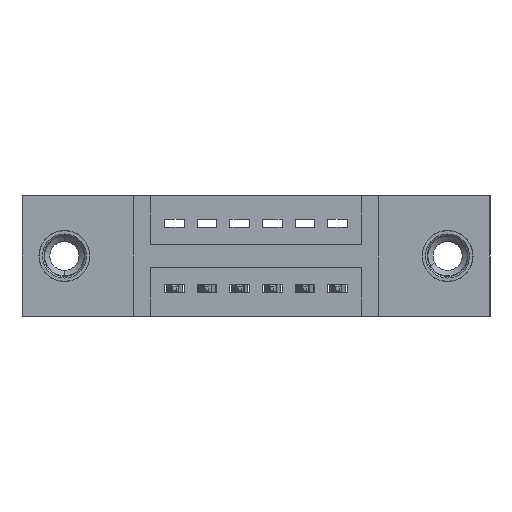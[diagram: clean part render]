
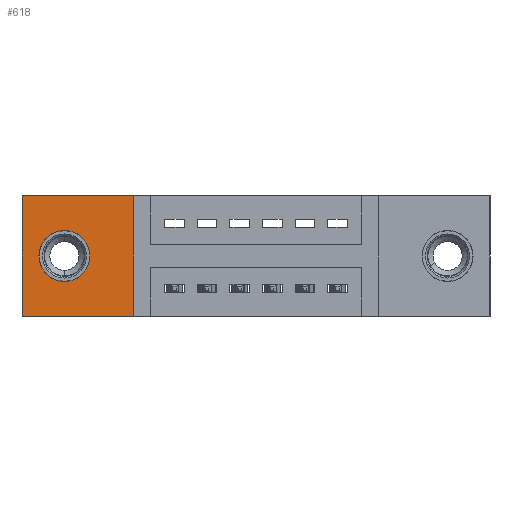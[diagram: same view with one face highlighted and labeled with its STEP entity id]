
A CAD part, front view. The second image highlights one B-rep face of the part: STEP entity #618.
In plain terms, the highlighted planar face has unit normal (0, -1, 0).
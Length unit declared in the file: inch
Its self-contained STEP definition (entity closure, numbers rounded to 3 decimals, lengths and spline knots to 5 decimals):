
#246 = EDGE_CURVE ( 'NONE', #9631, #3768, #4817, .T. ) ;
#498 = CARTESIAN_POINT ( 'NONE',  ( 0.3425, 0.11, 0. ) ) ;
#618 = ADVANCED_FACE ( 'NONE', ( #880, #6588 ), #7537, .T. ) ;
#830 = CARTESIAN_POINT ( 'NONE',  ( 0., 0.11, 0. ) ) ;
#880 = FACE_BOUND ( 'NONE', #8370, .T. ) ;
#921 = DIRECTION ( 'NONE',  ( -1., 0., 0. ) ) ;
#964 = ORIENTED_EDGE ( 'NONE', *, *, #3674, .T. ) ;
#1042 = CARTESIAN_POINT ( 'NONE',  ( 0.3425, 0.11, -0.37 ) ) ;
#1269 = CARTESIAN_POINT ( 'NONE',  ( 0.13, 0.11, -0.185 ) ) ;
#1862 = DIRECTION ( 'NONE',  ( 0., 0., -1. ) ) ;
#2298 = ORIENTED_EDGE ( 'NONE', *, *, #6666, .T. ) ;
#2589 = CARTESIAN_POINT ( 'NONE',  ( 0., 0.11, -0.37 ) ) ;
#2631 = EDGE_CURVE ( 'NONE', #8659, #7389, #10583, .T. ) ;
#2839 = VECTOR ( 'NONE', #921, 39.37008 ) ;
#2931 = DIRECTION ( 'NONE',  ( 0., -1., 0. ) ) ;
#3047 = DIRECTION ( 'NONE',  ( 0., -1., 0. ) ) ;
#3279 = CARTESIAN_POINT ( 'NONE',  ( 0.3425, 0.11, 0. ) ) ;
#3674 = EDGE_CURVE ( 'NONE', #3768, #7413, #7433, .T. ) ;
#3762 = CARTESIAN_POINT ( 'NONE',  ( 0., 0.11, -0.37 ) ) ;
#3768 = VERTEX_POINT ( 'NONE', #830 ) ;
#3857 = VECTOR ( 'NONE', #5739, 39.37008 ) ;
#3947 = ORIENTED_EDGE ( 'NONE', *, *, #7594, .T. ) ;
#4101 = AXIS2_PLACEMENT_3D ( 'NONE', #7179, #3047, #5514 ) ;
#4582 = DIRECTION ( 'NONE',  ( 0., 0., -1. ) ) ;
#4606 = AXIS2_PLACEMENT_3D ( 'NONE', #1269, #2931, #8740 ) ;
#4817 = LINE ( 'NONE', #9949, #2839 ) ;
#5016 = AXIS2_PLACEMENT_3D ( 'NONE', #2589, #7607, #1862 ) ;
#5181 = CARTESIAN_POINT ( 'NONE',  ( 0.13, 0.11, -0.263 ) ) ;
#5484 = CARTESIAN_POINT ( 'NONE',  ( 0., 0.11, 0. ) ) ;
#5514 = DIRECTION ( 'NONE',  ( 0., 0., -1. ) ) ;
#5739 = DIRECTION ( 'NONE',  ( 0., 0., 1. ) ) ;
#6056 = LINE ( 'NONE', #3279, #3857 ) ;
#6147 = VERTEX_POINT ( 'NONE', #1042 ) ;
#6248 = EDGE_CURVE ( 'NONE', #7389, #8659, #10251, .T. ) ;
#6408 = ORIENTED_EDGE ( 'NONE', *, *, #2631, .F. ) ;
#6459 = ORIENTED_EDGE ( 'NONE', *, *, #6248, .F. ) ;
#6588 = FACE_OUTER_BOUND ( 'NONE', #9590, .T. ) ;
#6596 = VECTOR ( 'NONE', #8569, 39.37008 ) ;
#6666 = EDGE_CURVE ( 'NONE', #7413, #6147, #8819, .T. ) ;
#6922 = CARTESIAN_POINT ( 'NONE',  ( 0., 0.11, -0.37 ) ) ;
#7179 = CARTESIAN_POINT ( 'NONE',  ( 0.13, 0.11, -0.185 ) ) ;
#7389 = VERTEX_POINT ( 'NONE', #10329 ) ;
#7413 = VERTEX_POINT ( 'NONE', #3762 ) ;
#7433 = LINE ( 'NONE', #5484, #9158 ) ;
#7537 = PLANE ( 'NONE',  #5016 ) ;
#7594 = EDGE_CURVE ( 'NONE', #6147, #9631, #6056, .T. ) ;
#7607 = DIRECTION ( 'NONE',  ( 0., -1., 0. ) ) ;
#8370 = EDGE_LOOP ( 'NONE', ( #6459, #6408 ) ) ;
#8569 = DIRECTION ( 'NONE',  ( 1., 0., 0. ) ) ;
#8590 = ORIENTED_EDGE ( 'NONE', *, *, #246, .T. ) ;
#8659 = VERTEX_POINT ( 'NONE', #5181 ) ;
#8740 = DIRECTION ( 'NONE',  ( 0., 0., -1. ) ) ;
#8819 = LINE ( 'NONE', #6922, #6596 ) ;
#9158 = VECTOR ( 'NONE', #4582, 39.37008 ) ;
#9590 = EDGE_LOOP ( 'NONE', ( #964, #2298, #3947, #8590 ) ) ;
#9631 = VERTEX_POINT ( 'NONE', #498 ) ;
#9949 = CARTESIAN_POINT ( 'NONE',  ( 0., 0.11, 0. ) ) ;
#10251 = CIRCLE ( 'NONE', #4606, 0.078 ) ;
#10329 = CARTESIAN_POINT ( 'NONE',  ( 0.13, 0.11, -0.107 ) ) ;
#10583 = CIRCLE ( 'NONE', #4101, 0.078 ) ;
